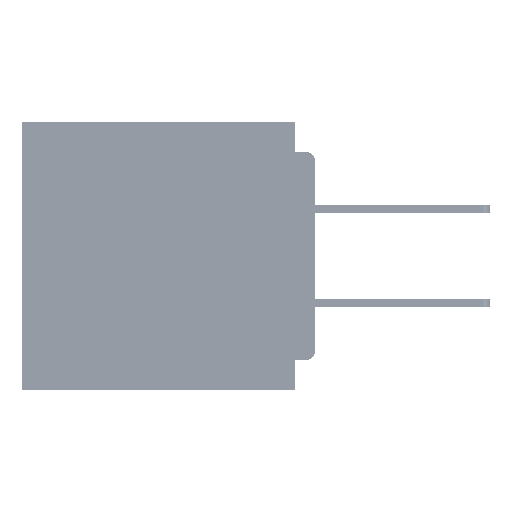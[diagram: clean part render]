
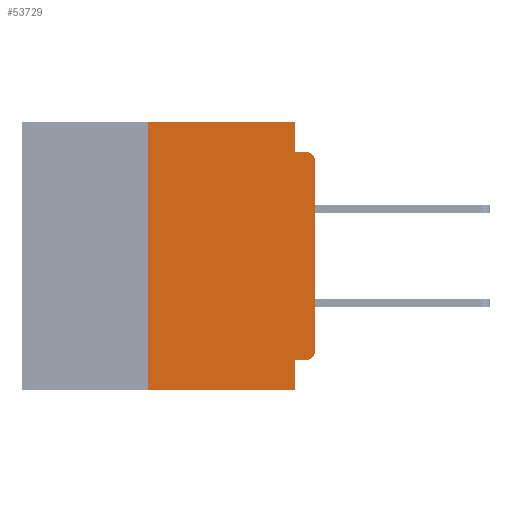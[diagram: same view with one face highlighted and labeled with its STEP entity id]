
A CAD part, left-side view. The second image highlights one B-rep face of the part: STEP entity #53729.
In plain terms, the highlighted planar face has unit normal (-1, 0, 0).
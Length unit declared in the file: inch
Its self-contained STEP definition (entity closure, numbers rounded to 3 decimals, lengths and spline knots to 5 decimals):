
#308 = CARTESIAN_POINT ( 'NONE',  ( 0., 0.25, -0.4 ) ) ;
#399 = VERTEX_POINT ( 'NONE', #9475 ) ;
#1748 = ORIENTED_EDGE ( 'NONE', *, *, #61020, .F. ) ;
#1876 = LINE ( 'NONE', #30095, #56283 ) ;
#2483 = DIRECTION ( 'NONE',  ( 0., 0., -1. ) ) ;
#3229 = ORIENTED_EDGE ( 'NONE', *, *, #58757, .F. ) ;
#3291 = ORIENTED_EDGE ( 'NONE', *, *, #42525, .F. ) ;
#3396 = DIRECTION ( 'NONE',  ( -1., 0., 0. ) ) ;
#3513 = EDGE_CURVE ( 'NONE', #41740, #40040, #16960, .T. ) ;
#3844 = DIRECTION ( 'NONE',  ( 0., -1., 0. ) ) ;
#4021 = CIRCLE ( 'NONE', #32806, 0.015 ) ;
#5061 = DIRECTION ( 'NONE',  ( 0., 0., -1. ) ) ;
#7296 = ORIENTED_EDGE ( 'NONE', *, *, #3513, .F. ) ;
#7656 = CARTESIAN_POINT ( 'NONE',  ( 0., 0.031, -0.045 ) ) ;
#8495 = VECTOR ( 'NONE', #51053, 39.37008 ) ;
#9475 = CARTESIAN_POINT ( 'NONE',  ( 0., 0.015, -0.355 ) ) ;
#9871 = CARTESIAN_POINT ( 'NONE',  ( 0., 0.031, 0. ) ) ;
#11940 = DIRECTION ( 'NONE',  ( 1., 0., 0. ) ) ;
#13481 = EDGE_CURVE ( 'NONE', #14117, #40040, #4021, .T. ) ;
#13586 = CARTESIAN_POINT ( 'NONE',  ( 0., 0.031, -0.355 ) ) ;
#13895 = DIRECTION ( 'NONE',  ( 0., -1., 0. ) ) ;
#14117 = VERTEX_POINT ( 'NONE', #63283 ) ;
#14686 = ORIENTED_EDGE ( 'NONE', *, *, #13481, .T. ) ;
#14773 = VERTEX_POINT ( 'NONE', #9871 ) ;
#14865 = AXIS2_PLACEMENT_3D ( 'NONE', #35923, #3396, #41408 ) ;
#15592 = DIRECTION ( 'NONE',  ( 0., 0., 1. ) ) ;
#16727 = EDGE_CURVE ( 'NONE', #62471, #14117, #22894, .T. ) ;
#16960 = LINE ( 'NONE', #36371, #58584 ) ;
#18675 = EDGE_CURVE ( 'NONE', #31418, #65166, #68408, .T. ) ;
#19124 = LINE ( 'NONE', #37578, #62458 ) ;
#19352 = ORIENTED_EDGE ( 'NONE', *, *, #18675, .F. ) ;
#19941 = DIRECTION ( 'NONE',  ( -1., 0., 0. ) ) ;
#22894 = LINE ( 'NONE', #29243, #8495 ) ;
#25892 = CARTESIAN_POINT ( 'NONE',  ( 0., 0., -0.34 ) ) ;
#29243 = CARTESIAN_POINT ( 'NONE',  ( 0., 0., 0. ) ) ;
#29861 = EDGE_LOOP ( 'NONE', ( #32674, #14686, #7296, #1748, #3291, #3229, #45711, #19352, #50056, #65316 ) ) ;
#30095 = CARTESIAN_POINT ( 'NONE',  ( 0., 0.437, 0. ) ) ;
#31418 = VERTEX_POINT ( 'NONE', #13586 ) ;
#32674 = ORIENTED_EDGE ( 'NONE', *, *, #16727, .T. ) ;
#32806 = AXIS2_PLACEMENT_3D ( 'NONE', #52477, #19941, #57949 ) ;
#33515 = PLANE ( 'NONE',  #52337 ) ;
#34839 = CARTESIAN_POINT ( 'NONE',  ( 0., 0.437, -0.4 ) ) ;
#35923 = CARTESIAN_POINT ( 'NONE',  ( 0., 0.015, -0.34 ) ) ;
#36371 = CARTESIAN_POINT ( 'NONE',  ( 0., 0., -0.045 ) ) ;
#37372 = DIRECTION ( 'NONE',  ( 0., 1., 0. ) ) ;
#37578 = CARTESIAN_POINT ( 'NONE',  ( 0., 0.031, 0. ) ) ;
#39716 = CARTESIAN_POINT ( 'NONE',  ( 0., 0.031, -0.4 ) ) ;
#40040 = VERTEX_POINT ( 'NONE', #48403 ) ;
#41107 = CARTESIAN_POINT ( 'NONE',  ( 0., 0.25, 0. ) ) ;
#41408 = DIRECTION ( 'NONE',  ( 0., 0., -1. ) ) ;
#41740 = VERTEX_POINT ( 'NONE', #7656 ) ;
#42525 = EDGE_CURVE ( 'NONE', #62351, #14773, #1876, .T. ) ;
#43480 = FACE_OUTER_BOUND ( 'NONE', #29861, .T. ) ;
#44200 = EDGE_CURVE ( 'NONE', #60441, #65166, #62050, .T. ) ;
#45711 = ORIENTED_EDGE ( 'NONE', *, *, #44200, .T. ) ;
#48403 = CARTESIAN_POINT ( 'NONE',  ( 0., 0.015, -0.045 ) ) ;
#49932 = DIRECTION ( 'NONE',  ( 0., 0., -1. ) ) ;
#50056 = ORIENTED_EDGE ( 'NONE', *, *, #53536, .F. ) ;
#51053 = DIRECTION ( 'NONE',  ( 0., 0., 1. ) ) ;
#51241 = EDGE_CURVE ( 'NONE', #399, #62471, #65010, .T. ) ;
#52334 = VECTOR ( 'NONE', #2483, 39.37008 ) ;
#52337 = AXIS2_PLACEMENT_3D ( 'NONE', #60596, #11940, #49932 ) ;
#52477 = CARTESIAN_POINT ( 'NONE',  ( 0., 0.015, -0.06 ) ) ;
#53333 = CARTESIAN_POINT ( 'NONE',  ( 0., 0.25, -0.4 ) ) ;
#53536 = EDGE_CURVE ( 'NONE', #399, #31418, #68779, .T. ) ;
#53729 = ADVANCED_FACE ( 'NONE', ( #43480 ), #33515, .F. ) ;
#54431 = VECTOR ( 'NONE', #37372, 39.37008 ) ;
#56283 = VECTOR ( 'NONE', #13895, 39.37008 ) ;
#57949 = DIRECTION ( 'NONE',  ( 0., 0., -1. ) ) ;
#58584 = VECTOR ( 'NONE', #3844, 39.37008 ) ;
#58757 = EDGE_CURVE ( 'NONE', #60441, #62351, #67848, .T. ) ;
#60441 = VERTEX_POINT ( 'NONE', #308 ) ;
#60596 = CARTESIAN_POINT ( 'NONE',  ( 0., 0.437, 0. ) ) ;
#61020 = EDGE_CURVE ( 'NONE', #14773, #41740, #19124, .T. ) ;
#61886 = DIRECTION ( 'NONE',  ( 0., -1., 0. ) ) ;
#62050 = LINE ( 'NONE', #34839, #63732 ) ;
#62075 = CARTESIAN_POINT ( 'NONE',  ( 0., 0.031, -0.4 ) ) ;
#62351 = VERTEX_POINT ( 'NONE', #41107 ) ;
#62458 = VECTOR ( 'NONE', #5061, 39.37008 ) ;
#62471 = VERTEX_POINT ( 'NONE', #25892 ) ;
#63283 = CARTESIAN_POINT ( 'NONE',  ( 0., 0., -0.06 ) ) ;
#63732 = VECTOR ( 'NONE', #61886, 39.37008 ) ;
#64373 = CARTESIAN_POINT ( 'NONE',  ( 0., 0., -0.355 ) ) ;
#64472 = VECTOR ( 'NONE', #15592, 39.37008 ) ;
#65010 = CIRCLE ( 'NONE', #14865, 0.015 ) ;
#65166 = VERTEX_POINT ( 'NONE', #39716 ) ;
#65316 = ORIENTED_EDGE ( 'NONE', *, *, #51241, .T. ) ;
#67848 = LINE ( 'NONE', #53333, #64472 ) ;
#68408 = LINE ( 'NONE', #62075, #52334 ) ;
#68779 = LINE ( 'NONE', #64373, #54431 ) ;
